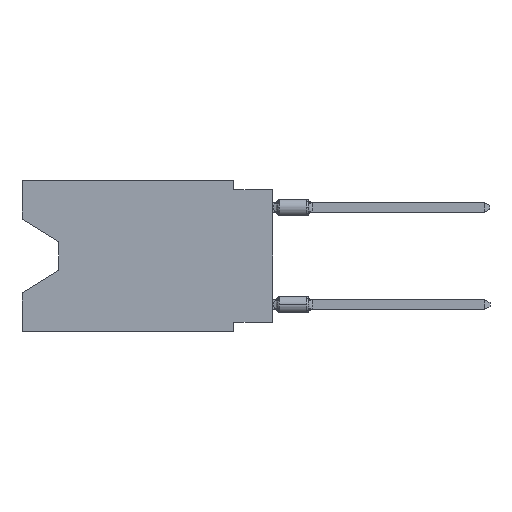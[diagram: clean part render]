
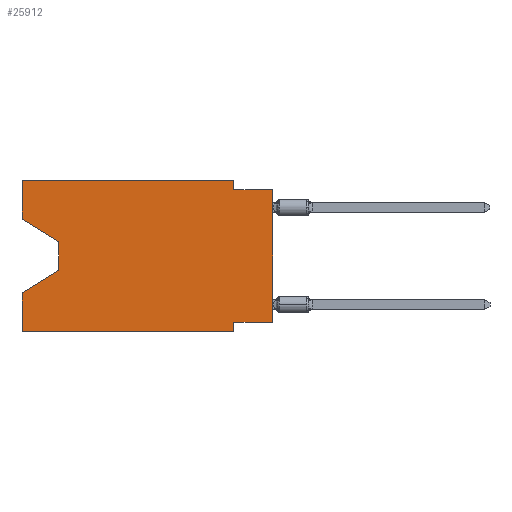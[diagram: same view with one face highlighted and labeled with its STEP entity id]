
A CAD part, left-side view. The second image highlights one B-rep face of the part: STEP entity #25912.
In plain terms, the highlighted planar face has unit normal (-1, 0, 0).
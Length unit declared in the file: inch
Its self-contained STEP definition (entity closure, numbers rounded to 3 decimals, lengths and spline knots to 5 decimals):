
#665 = DIRECTION ( 'NONE',  ( 0., -1., 0. ) ) ;
#2303 = VERTEX_POINT ( 'NONE', #51055 ) ;
#2481 = EDGE_CURVE ( 'NONE', #40449, #41080, #37538, .T. ) ;
#2512 = VECTOR ( 'NONE', #48736, 39.37008 ) ;
#3197 = CARTESIAN_POINT ( 'NONE',  ( 0., 0.1, 0. ) ) ;
#3425 = ORIENTED_EDGE ( 'NONE', *, *, #38352, .F. ) ;
#3765 = LINE ( 'NONE', #44203, #39944 ) ;
#4805 = VERTEX_POINT ( 'NONE', #5727 ) ;
#4834 = ORIENTED_EDGE ( 'NONE', *, *, #26804, .T. ) ;
#4903 = EDGE_CURVE ( 'NONE', #17159, #37487, #35016, .T. ) ;
#5058 = CARTESIAN_POINT ( 'NONE',  ( 0., 0.55, -0.232 ) ) ;
#5134 = EDGE_CURVE ( 'NONE', #17159, #41080, #28142, .T. ) ;
#5727 = CARTESIAN_POINT ( 'NONE',  ( 0., 0.645, 0. ) ) ;
#5896 = LINE ( 'NONE', #13818, #30723 ) ;
#6578 = DIRECTION ( 'NONE',  ( 0., -1., 0. ) ) ;
#6686 = CARTESIAN_POINT ( 'NONE',  ( 0., 0., -0.365 ) ) ;
#8227 = CARTESIAN_POINT ( 'NONE',  ( 0., 0.645, 0. ) ) ;
#8265 = DIRECTION ( 'NONE',  ( 0., 0., -1. ) ) ;
#8350 = DIRECTION ( 'NONE',  ( 0., 0., 1. ) ) ;
#8886 = VECTOR ( 'NONE', #665, 39.37008 ) ;
#9193 = CARTESIAN_POINT ( 'NONE',  ( 0., 0.1, -0.39 ) ) ;
#9252 = CARTESIAN_POINT ( 'NONE',  ( 0., 0.645, -0.10025 ) ) ;
#10546 = LINE ( 'NONE', #22186, #21076 ) ;
#11289 = VECTOR ( 'NONE', #20891, 39.37008 ) ;
#12120 = LINE ( 'NONE', #9193, #21224 ) ;
#12338 = LINE ( 'NONE', #16029, #40939 ) ;
#12597 = ORIENTED_EDGE ( 'NONE', *, *, #21043, .T. ) ;
#13818 = CARTESIAN_POINT ( 'NONE',  ( 0., 0., 0. ) ) ;
#15246 = VERTEX_POINT ( 'NONE', #32411 ) ;
#15454 = DIRECTION ( 'NONE',  ( 0., -1., 0. ) ) ;
#15458 = LINE ( 'NONE', #31576, #16091 ) ;
#15901 = ORIENTED_EDGE ( 'NONE', *, *, #5134, .F. ) ;
#16029 = CARTESIAN_POINT ( 'NONE',  ( 0., 0.645, 0. ) ) ;
#16091 = VECTOR ( 'NONE', #47706, 39.37008 ) ;
#16149 = PLANE ( 'NONE',  #50069 ) ;
#16424 = ORIENTED_EDGE ( 'NONE', *, *, #32887, .F. ) ;
#16853 = EDGE_CURVE ( 'NONE', #47049, #23071, #15458, .T. ) ;
#17123 = DIRECTION ( 'NONE',  ( 0., 0., -1. ) ) ;
#17159 = VERTEX_POINT ( 'NONE', #31979 ) ;
#18217 = ORIENTED_EDGE ( 'NONE', *, *, #4903, .T. ) ;
#19054 = ORIENTED_EDGE ( 'NONE', *, *, #36810, .T. ) ;
#20556 = CARTESIAN_POINT ( 'NONE',  ( 0., 0., -0.365 ) ) ;
#20891 = DIRECTION ( 'NONE',  ( 0., -0.855, -0.519 ) ) ;
#21032 = CARTESIAN_POINT ( 'NONE',  ( 0., 0.645, 0. ) ) ;
#21043 = EDGE_CURVE ( 'NONE', #40220, #40449, #3765, .T. ) ;
#21076 = VECTOR ( 'NONE', #6578, 39.37008 ) ;
#21224 = VECTOR ( 'NONE', #17123, 39.37008 ) ;
#22186 = CARTESIAN_POINT ( 'NONE',  ( 0., 0., -0.025 ) ) ;
#23071 = VERTEX_POINT ( 'NONE', #47019 ) ;
#23401 = CARTESIAN_POINT ( 'NONE',  ( 0., 0.645, -0.39 ) ) ;
#25912 = ADVANCED_FACE ( 'NONE', ( #36218 ), #16149, .F. ) ;
#26215 = EDGE_LOOP ( 'NONE', ( #19054, #12597, #27513, #15901, #18217, #32115, #16424, #4834, #45220, #44073, #3425, #43518 ) ) ;
#26804 = EDGE_CURVE ( 'NONE', #40112, #2303, #5896, .T. ) ;
#27045 = VECTOR ( 'NONE', #15454, 39.37008 ) ;
#27399 = CARTESIAN_POINT ( 'NONE',  ( 0., 0.645, -0.10025 ) ) ;
#27513 = ORIENTED_EDGE ( 'NONE', *, *, #2481, .T. ) ;
#27874 = EDGE_CURVE ( 'NONE', #51467, #4805, #12338, .T. ) ;
#28142 = LINE ( 'NONE', #32615, #2512 ) ;
#28829 = DIRECTION ( 'NONE',  ( 0., 0.855, -0.519 ) ) ;
#30236 = EDGE_CURVE ( 'NONE', #23071, #2303, #10546, .T. ) ;
#30723 = VECTOR ( 'NONE', #8350, 39.37008 ) ;
#31576 = CARTESIAN_POINT ( 'NONE',  ( 0., 0.1, 0. ) ) ;
#31749 = DIRECTION ( 'NONE',  ( 0., 0., -1. ) ) ;
#31928 = DIRECTION ( 'NONE',  ( 0., 1., 0. ) ) ;
#31979 = CARTESIAN_POINT ( 'NONE',  ( 0., 0.645, -0.39 ) ) ;
#32115 = ORIENTED_EDGE ( 'NONE', *, *, #51261, .F. ) ;
#32411 = CARTESIAN_POINT ( 'NONE',  ( 0., 0.1, -0.365 ) ) ;
#32614 = CARTESIAN_POINT ( 'NONE',  ( 0., 0.645, -0.28975 ) ) ;
#32615 = CARTESIAN_POINT ( 'NONE',  ( 0., 0.645, 0. ) ) ;
#32887 = EDGE_CURVE ( 'NONE', #40112, #15246, #39853, .T. ) ;
#33814 = VECTOR ( 'NONE', #31928, 39.37008 ) ;
#35016 = LINE ( 'NONE', #23401, #27045 ) ;
#36218 = FACE_OUTER_BOUND ( 'NONE', #26215, .T. ) ;
#36810 = EDGE_CURVE ( 'NONE', #51467, #40220, #40968, .T. ) ;
#37009 = CARTESIAN_POINT ( 'NONE',  ( 0., 0.55, -0.232 ) ) ;
#37487 = VERTEX_POINT ( 'NONE', #45465 ) ;
#37538 = LINE ( 'NONE', #37009, #42001 ) ;
#38352 = EDGE_CURVE ( 'NONE', #4805, #47049, #40838, .T. ) ;
#39853 = LINE ( 'NONE', #20556, #33814 ) ;
#39944 = VECTOR ( 'NONE', #8265, 39.37008 ) ;
#40112 = VERTEX_POINT ( 'NONE', #6686 ) ;
#40220 = VERTEX_POINT ( 'NONE', #48399 ) ;
#40449 = VERTEX_POINT ( 'NONE', #5058 ) ;
#40838 = LINE ( 'NONE', #21032, #8886 ) ;
#40939 = VECTOR ( 'NONE', #51965, 39.37008 ) ;
#40968 = LINE ( 'NONE', #9252, #11289 ) ;
#41080 = VERTEX_POINT ( 'NONE', #32614 ) ;
#42001 = VECTOR ( 'NONE', #28829, 39.37008 ) ;
#43518 = ORIENTED_EDGE ( 'NONE', *, *, #27874, .F. ) ;
#44073 = ORIENTED_EDGE ( 'NONE', *, *, #16853, .F. ) ;
#44203 = CARTESIAN_POINT ( 'NONE',  ( 0., 0.55, -0.158 ) ) ;
#45220 = ORIENTED_EDGE ( 'NONE', *, *, #30236, .F. ) ;
#45465 = CARTESIAN_POINT ( 'NONE',  ( 0., 0.1, -0.39 ) ) ;
#47019 = CARTESIAN_POINT ( 'NONE',  ( 0., 0.1, -0.025 ) ) ;
#47049 = VERTEX_POINT ( 'NONE', #3197 ) ;
#47706 = DIRECTION ( 'NONE',  ( 0., 0., -1. ) ) ;
#48399 = CARTESIAN_POINT ( 'NONE',  ( 0., 0.55, -0.158 ) ) ;
#48736 = DIRECTION ( 'NONE',  ( 0., 0., 1. ) ) ;
#48893 = DIRECTION ( 'NONE',  ( 1., 0., 0. ) ) ;
#50069 = AXIS2_PLACEMENT_3D ( 'NONE', #8227, #48893, #31749 ) ;
#51055 = CARTESIAN_POINT ( 'NONE',  ( 0., 0., -0.025 ) ) ;
#51261 = EDGE_CURVE ( 'NONE', #15246, #37487, #12120, .T. ) ;
#51467 = VERTEX_POINT ( 'NONE', #27399 ) ;
#51965 = DIRECTION ( 'NONE',  ( 0., 0., 1. ) ) ;
